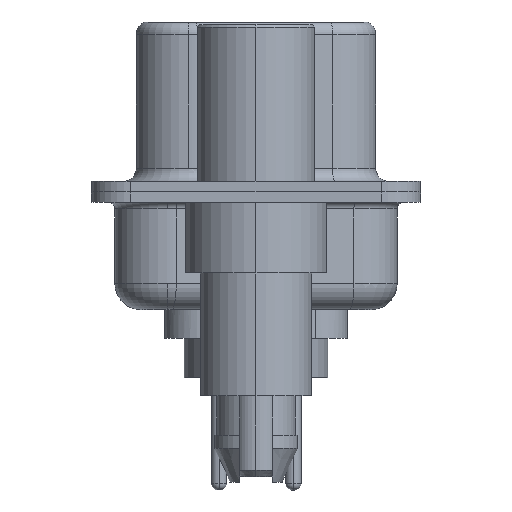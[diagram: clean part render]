
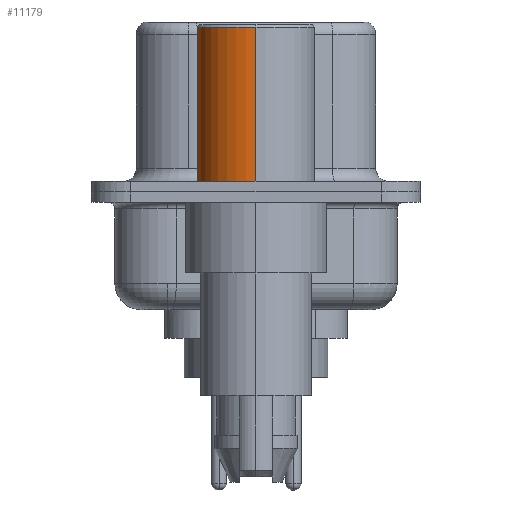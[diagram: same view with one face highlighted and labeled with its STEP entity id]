
A CAD part, left-side view. The second image highlights one B-rep face of the part: STEP entity #11179.
In plain terms, the highlighted cylindrical face has radius 2.25 mm (diameter 4.5 mm), a partial arc.
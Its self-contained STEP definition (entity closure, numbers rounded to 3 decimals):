
#251 = ORIENTED_EDGE ( 'NONE', *, *, #10609, .F. ) ;
#508 = CARTESIAN_POINT ( 'NONE',  ( 2.25, 0., 0.4 ) ) ;
#1033 = DIRECTION ( 'NONE',  ( 1., 0., 0. ) ) ;
#1244 = EDGE_CURVE ( 'NONE', #9071, #11362, #8254, .T. ) ;
#2033 = CARTESIAN_POINT ( 'NONE',  ( 0., 0., 6.3 ) ) ;
#2242 = AXIS2_PLACEMENT_3D ( 'NONE', #13447, #8496, #1033 ) ;
#2602 = DIRECTION ( 'NONE',  ( 0., 0., 1. ) ) ;
#2938 = ORIENTED_EDGE ( 'NONE', *, *, #1244, .F. ) ;
#3246 = CARTESIAN_POINT ( 'NONE',  ( 2.25, 0., 6.3 ) ) ;
#3249 = DIRECTION ( 'NONE',  ( 1., 0., 0. ) ) ;
#3511 = CYLINDRICAL_SURFACE ( 'NONE', #2242, 2.25 ) ;
#4500 = AXIS2_PLACEMENT_3D ( 'NONE', #10071, #2602, #11306 ) ;
#7140 = ORIENTED_EDGE ( 'NONE', *, *, #15143, .T. ) ;
#7894 = VERTEX_POINT ( 'NONE', #9547 ) ;
#8192 = DIRECTION ( 'NONE',  ( 0., 0., 1. ) ) ;
#8244 = CARTESIAN_POINT ( 'NONE',  ( 2.25, 0., 0.581 ) ) ;
#8254 = LINE ( 'NONE', #8244, #11579 ) ;
#8496 = DIRECTION ( 'NONE',  ( 0., 0., 1. ) ) ;
#8757 = CIRCLE ( 'NONE', #4500, 2.25 ) ;
#9071 = VERTEX_POINT ( 'NONE', #508 ) ;
#9547 = CARTESIAN_POINT ( 'NONE',  ( -2.25, 0., 6.3 ) ) ;
#10071 = CARTESIAN_POINT ( 'NONE',  ( 0., 0., 0.4 ) ) ;
#10609 = EDGE_CURVE ( 'NONE', #11362, #7894, #15058, .T. ) ;
#10716 = DIRECTION ( 'NONE',  ( 0., 0., 1. ) ) ;
#11179 = ADVANCED_FACE ( 'NONE', ( #13819 ), #3511, .T. ) ;
#11306 = DIRECTION ( 'NONE',  ( 1., 0., 0. ) ) ;
#11362 = VERTEX_POINT ( 'NONE', #3246 ) ;
#11557 = VERTEX_POINT ( 'NONE', #12270 ) ;
#11572 = AXIS2_PLACEMENT_3D ( 'NONE', #2033, #10716, #3249 ) ;
#11579 = VECTOR ( 'NONE', #8192, 1000. ) ;
#11863 = CARTESIAN_POINT ( 'NONE',  ( -2.25, 0., 0.581 ) ) ;
#12053 = VECTOR ( 'NONE', #14351, 1000. ) ;
#12270 = CARTESIAN_POINT ( 'NONE',  ( -2.25, 0., 0.4 ) ) ;
#12974 = EDGE_CURVE ( 'NONE', #9071, #11557, #8757, .T. ) ;
#13441 = EDGE_LOOP ( 'NONE', ( #14628, #7140, #251, #2938 ) ) ;
#13447 = CARTESIAN_POINT ( 'NONE',  ( 0., 0., 0.581 ) ) ;
#13819 = FACE_OUTER_BOUND ( 'NONE', #13441, .T. ) ;
#14351 = DIRECTION ( 'NONE',  ( 0., 0., 1. ) ) ;
#14628 = ORIENTED_EDGE ( 'NONE', *, *, #12974, .T. ) ;
#15058 = CIRCLE ( 'NONE', #11572, 2.25 ) ;
#15143 = EDGE_CURVE ( 'NONE', #11557, #7894, #15705, .T. ) ;
#15705 = LINE ( 'NONE', #11863, #12053 ) ;
